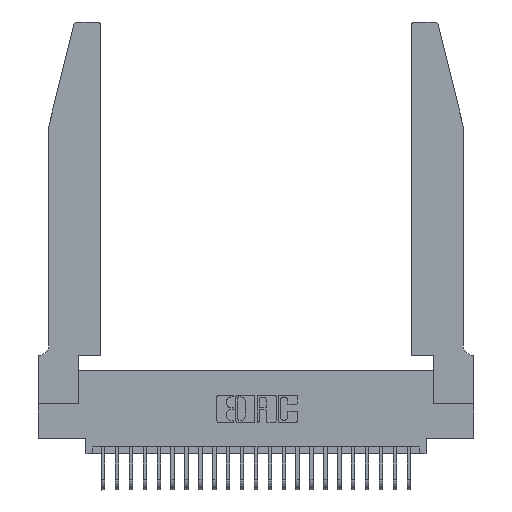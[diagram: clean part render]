
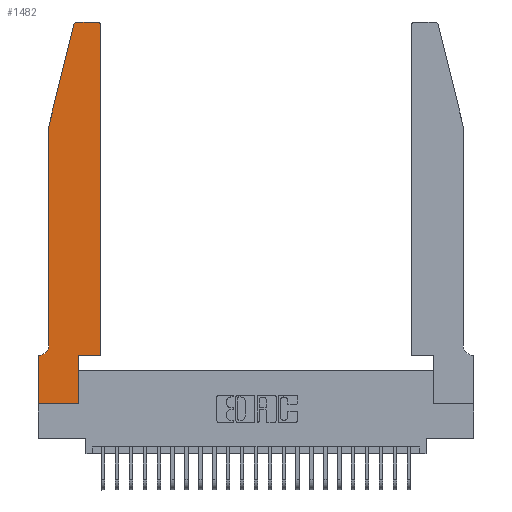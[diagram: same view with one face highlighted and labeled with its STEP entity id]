
A CAD part, top view. The second image highlights one B-rep face of the part: STEP entity #1482.
In plain terms, the highlighted planar face has unit normal (0, 0, 1).
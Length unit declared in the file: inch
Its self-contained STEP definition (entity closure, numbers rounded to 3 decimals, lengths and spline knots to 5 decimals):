
#13 = DIRECTION ( 'NONE',  ( 0., 0., 1. ) ) ;
#59 = FACE_OUTER_BOUND ( 'NONE', #13227, .T. ) ;
#510 = DIRECTION ( 'NONE',  ( 1., 0., 0. ) ) ;
#744 = DIRECTION ( 'NONE',  ( 0., 0., -1. ) ) ;
#1482 = ADVANCED_FACE ( 'NONE', ( #59 ), #20801, .T. ) ;
#1730 = VERTEX_POINT ( 'NONE', #21973 ) ;
#1846 = AXIS2_PLACEMENT_3D ( 'NONE', #23480, #12027, #510 ) ;
#2730 = VERTEX_POINT ( 'NONE', #7246 ) ;
#3014 = ORIENTED_EDGE ( 'NONE', *, *, #4436, .T. ) ;
#3340 = EDGE_CURVE ( 'NONE', #18729, #8060, #14691, .T. ) ;
#3859 = EDGE_CURVE ( 'NONE', #1730, #23859, #23047, .T. ) ;
#4436 = EDGE_CURVE ( 'NONE', #12149, #17447, #16116, .T. ) ;
#5016 = LINE ( 'NONE', #15163, #24741 ) ;
#5106 = ORIENTED_EDGE ( 'NONE', *, *, #14265, .T. ) ;
#5135 = CARTESIAN_POINT ( 'NONE',  ( 0.0055, 0.35, 0.37 ) ) ;
#5863 = VERTEX_POINT ( 'NONE', #6184 ) ;
#6167 = AXIS2_PLACEMENT_3D ( 'NONE', #12250, #744, #14164 ) ;
#6184 = CARTESIAN_POINT ( 'NONE',  ( 0., 0., 0.37 ) ) ;
#6287 = EDGE_CURVE ( 'NONE', #23901, #1730, #5016, .T. ) ;
#6309 = ORIENTED_EDGE ( 'NONE', *, *, #11187, .T. ) ;
#6971 = LINE ( 'NONE', #7937, #23701 ) ;
#7069 = ORIENTED_EDGE ( 'NONE', *, *, #15618, .T. ) ;
#7089 = CARTESIAN_POINT ( 'NONE',  ( 0.0755, 2., 0.37 ) ) ;
#7246 = CARTESIAN_POINT ( 'NONE',  ( 0.284, 2.75, 0.37 ) ) ;
#7800 = VECTOR ( 'NONE', #14280, 39.37008 ) ;
#7937 = CARTESIAN_POINT ( 'NONE',  ( 0.2865, 0.35, 0.37 ) ) ;
#8060 = VERTEX_POINT ( 'NONE', #8966 ) ;
#8574 = CARTESIAN_POINT ( 'NONE',  ( 0.0755, 0.42, 0.37 ) ) ;
#8608 = CARTESIAN_POINT ( 'NONE',  ( 0., 0., 0.37 ) ) ;
#8966 = CARTESIAN_POINT ( 'NONE',  ( 0.0755, 2., 0.37 ) ) ;
#8970 = DIRECTION ( 'NONE',  ( 0., -1., 0. ) ) ;
#9062 = LINE ( 'NONE', #8608, #9669 ) ;
#9119 = ORIENTED_EDGE ( 'NONE', *, *, #15228, .T. ) ;
#9166 = DIRECTION ( 'NONE',  ( 1., 0., 0. ) ) ;
#9208 = AXIS2_PLACEMENT_3D ( 'NONE', #11559, #13, #13456 ) ;
#9593 = VECTOR ( 'NONE', #15203, 39.37008 ) ;
#9669 = VECTOR ( 'NONE', #20044, 39.37008 ) ;
#9864 = DIRECTION ( 'NONE',  ( 0., 1., 0. ) ) ;
#10140 = CARTESIAN_POINT ( 'NONE',  ( 0.4505, 2.72, 0.37 ) ) ;
#10159 = VECTOR ( 'NONE', #11350, 39.37008 ) ;
#10222 = VECTOR ( 'NONE', #10900, 39.37008 ) ;
#10900 = DIRECTION ( 'NONE',  ( -0.239, -0.971, 0. ) ) ;
#11187 = EDGE_CURVE ( 'NONE', #23859, #13973, #12342, .T. ) ;
#11350 = DIRECTION ( 'NONE',  ( 0., -1., 0. ) ) ;
#11449 = CIRCLE ( 'NONE', #1846, 0.03 ) ;
#11523 = CARTESIAN_POINT ( 'NONE',  ( 0.2605, 2.75, 0.37 ) ) ;
#11559 = CARTESIAN_POINT ( 'NONE',  ( 0.4205, 2.72, 0.37 ) ) ;
#11682 = CARTESIAN_POINT ( 'NONE',  ( 0., 0.35, 0.37 ) ) ;
#11845 = LINE ( 'NONE', #11523, #16294 ) ;
#12027 = DIRECTION ( 'NONE',  ( 0., 0., 1. ) ) ;
#12149 = VERTEX_POINT ( 'NONE', #8574 ) ;
#12250 = CARTESIAN_POINT ( 'NONE',  ( 0.0055, 0.42, 0.37 ) ) ;
#12342 = CIRCLE ( 'NONE', #9208, 0.03 ) ;
#12365 = CARTESIAN_POINT ( 'NONE',  ( 0.4505, 0.35, 0.37 ) ) ;
#13030 = VERTEX_POINT ( 'NONE', #11682 ) ;
#13227 = EDGE_LOOP ( 'NONE', ( #14108, #5106, #15224, #15517, #3014, #9119, #7069, #15676, #16891, #14953, #22782, #6309 ) ) ;
#13338 = DIRECTION ( 'NONE',  ( 1., 0., 0. ) ) ;
#13456 = DIRECTION ( 'NONE',  ( 1., 0., 0. ) ) ;
#13884 = EDGE_CURVE ( 'NONE', #5863, #15245, #9062, .T. ) ;
#13973 = VERTEX_POINT ( 'NONE', #20296 ) ;
#14108 = ORIENTED_EDGE ( 'NONE', *, *, #20771, .T. ) ;
#14164 = DIRECTION ( 'NONE',  ( -1., 0., 0. ) ) ;
#14192 = DIRECTION ( 'NONE',  ( 0., 0., 1. ) ) ;
#14265 = EDGE_CURVE ( 'NONE', #2730, #18729, #11449, .T. ) ;
#14280 = DIRECTION ( 'NONE',  ( 0., 1., 0. ) ) ;
#14691 = LINE ( 'NONE', #22335, #10222 ) ;
#14953 = ORIENTED_EDGE ( 'NONE', *, *, #6287, .T. ) ;
#15163 = CARTESIAN_POINT ( 'NONE',  ( 0.4505, 0.35, 0.37 ) ) ;
#15203 = DIRECTION ( 'NONE',  ( -1., 0., 0. ) ) ;
#15224 = ORIENTED_EDGE ( 'NONE', *, *, #3340, .T. ) ;
#15228 = EDGE_CURVE ( 'NONE', #17447, #13030, #24824, .T. ) ;
#15245 = VERTEX_POINT ( 'NONE', #19136 ) ;
#15517 = ORIENTED_EDGE ( 'NONE', *, *, #21698, .T. ) ;
#15546 = AXIS2_PLACEMENT_3D ( 'NONE', #20863, #14192, #9166 ) ;
#15618 = EDGE_CURVE ( 'NONE', #13030, #5863, #15812, .T. ) ;
#15676 = ORIENTED_EDGE ( 'NONE', *, *, #13884, .T. ) ;
#15812 = LINE ( 'NONE', #17084, #10159 ) ;
#16116 = CIRCLE ( 'NONE', #6167, 0.07 ) ;
#16252 = VECTOR ( 'NONE', #8970, 39.37008 ) ;
#16294 = VECTOR ( 'NONE', #23427, 39.37008 ) ;
#16842 = LINE ( 'NONE', #7089, #16252 ) ;
#16891 = ORIENTED_EDGE ( 'NONE', *, *, #22506, .T. ) ;
#17084 = CARTESIAN_POINT ( 'NONE',  ( 0., 0., 0.37 ) ) ;
#17447 = VERTEX_POINT ( 'NONE', #5135 ) ;
#17896 = CARTESIAN_POINT ( 'NONE',  ( 0.2865, 0.35, 0.37 ) ) ;
#18703 = CARTESIAN_POINT ( 'NONE',  ( 0.25487, 2.72718, 0.37 ) ) ;
#18729 = VERTEX_POINT ( 'NONE', #18703 ) ;
#19049 = CARTESIAN_POINT ( 'NONE',  ( 0.0755, 0.35, 0.37 ) ) ;
#19136 = CARTESIAN_POINT ( 'NONE',  ( 0.2865, 0., 0.37 ) ) ;
#20044 = DIRECTION ( 'NONE',  ( 1., 0., 0. ) ) ;
#20296 = CARTESIAN_POINT ( 'NONE',  ( 0.4205, 2.75, 0.37 ) ) ;
#20771 = EDGE_CURVE ( 'NONE', #13973, #2730, #11845, .T. ) ;
#20801 = PLANE ( 'NONE',  #15546 ) ;
#20863 = CARTESIAN_POINT ( 'NONE',  ( 0., 0.35, 0.37 ) ) ;
#21698 = EDGE_CURVE ( 'NONE', #8060, #12149, #16842, .T. ) ;
#21973 = CARTESIAN_POINT ( 'NONE',  ( 0.4505, 0.35, 0.37 ) ) ;
#22335 = CARTESIAN_POINT ( 'NONE',  ( 0.0755, 2., 0.37 ) ) ;
#22506 = EDGE_CURVE ( 'NONE', #15245, #23901, #6971, .T. ) ;
#22782 = ORIENTED_EDGE ( 'NONE', *, *, #3859, .T. ) ;
#23047 = LINE ( 'NONE', #12365, #7800 ) ;
#23427 = DIRECTION ( 'NONE',  ( -1., 0., 0. ) ) ;
#23480 = CARTESIAN_POINT ( 'NONE',  ( 0.284, 2.72, 0.37 ) ) ;
#23701 = VECTOR ( 'NONE', #9864, 39.37008 ) ;
#23859 = VERTEX_POINT ( 'NONE', #10140 ) ;
#23901 = VERTEX_POINT ( 'NONE', #17896 ) ;
#24741 = VECTOR ( 'NONE', #13338, 39.37008 ) ;
#24824 = LINE ( 'NONE', #19049, #9593 ) ;
